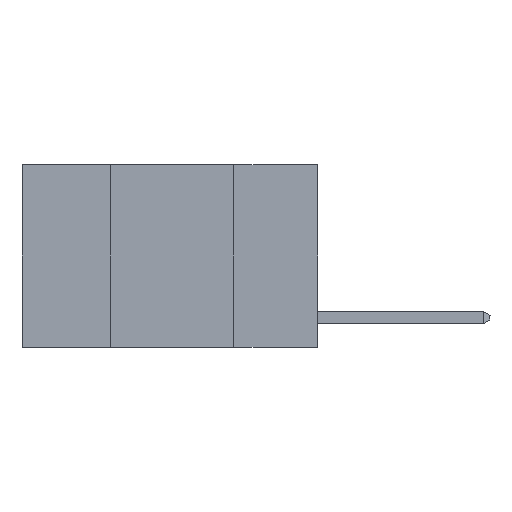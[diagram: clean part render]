
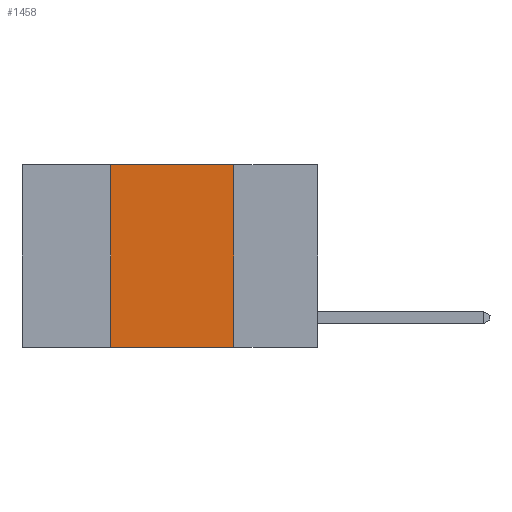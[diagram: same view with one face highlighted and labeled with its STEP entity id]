
A CAD part, left-side view. The second image highlights one B-rep face of the part: STEP entity #1458.
In plain terms, the highlighted planar face has unit normal (-1, 0, 0).
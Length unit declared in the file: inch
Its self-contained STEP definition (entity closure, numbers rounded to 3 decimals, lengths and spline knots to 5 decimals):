
#88 = LINE ( 'NONE', #13761, #22506 ) ;
#512 = VERTEX_POINT ( 'NONE', #4014 ) ;
#1458 = ADVANCED_FACE ( 'NONE', ( #5654 ), #13748, .F. ) ;
#1554 = DIRECTION ( 'NONE',  ( 0., 0., 1. ) ) ;
#3125 = EDGE_CURVE ( 'NONE', #16764, #26114, #20936, .T. ) ;
#3681 = DIRECTION ( 'NONE',  ( 0., -1., 0. ) ) ;
#4014 = CARTESIAN_POINT ( 'NONE',  ( 0., 0.42, -0.37 ) ) ;
#5654 = FACE_OUTER_BOUND ( 'NONE', #11573, .T. ) ;
#6169 = CARTESIAN_POINT ( 'NONE',  ( 0., 0.6, 0. ) ) ;
#6797 = EDGE_CURVE ( 'NONE', #25170, #16764, #20946, .T. ) ;
#6810 = DIRECTION ( 'NONE',  ( 1., 0., 0. ) ) ;
#7397 = CARTESIAN_POINT ( 'NONE',  ( 0., 0.17, -0.37 ) ) ;
#7670 = ORIENTED_EDGE ( 'NONE', *, *, #6797, .F. ) ;
#7905 = LINE ( 'NONE', #8155, #15253 ) ;
#8155 = CARTESIAN_POINT ( 'NONE',  ( 0., 0.42, 0. ) ) ;
#11036 = CARTESIAN_POINT ( 'NONE',  ( 0., 0.6, 0. ) ) ;
#11573 = EDGE_LOOP ( 'NONE', ( #22720, #7670, #16986, #24437 ) ) ;
#12397 = DIRECTION ( 'NONE',  ( 0., 0., -1. ) ) ;
#13748 = PLANE ( 'NONE',  #19317 ) ;
#13761 = CARTESIAN_POINT ( 'NONE',  ( 0., 0.6, -0.37 ) ) ;
#13836 = CARTESIAN_POINT ( 'NONE',  ( 0., 0.42, 0. ) ) ;
#14168 = EDGE_CURVE ( 'NONE', #512, #25170, #7905, .T. ) ;
#15253 = VECTOR ( 'NONE', #1554, 39.37008 ) ;
#16237 = VECTOR ( 'NONE', #25450, 39.37008 ) ;
#16619 = VECTOR ( 'NONE', #22917, 39.37008 ) ;
#16764 = VERTEX_POINT ( 'NONE', #24000 ) ;
#16981 = CARTESIAN_POINT ( 'NONE',  ( 0., 0.17, 0. ) ) ;
#16986 = ORIENTED_EDGE ( 'NONE', *, *, #14168, .F. ) ;
#19056 = EDGE_CURVE ( 'NONE', #512, #26114, #88, .T. ) ;
#19317 = AXIS2_PLACEMENT_3D ( 'NONE', #6169, #6810, #12397 ) ;
#20936 = LINE ( 'NONE', #16981, #16619 ) ;
#20946 = LINE ( 'NONE', #11036, #16237 ) ;
#22506 = VECTOR ( 'NONE', #3681, 39.37008 ) ;
#22720 = ORIENTED_EDGE ( 'NONE', *, *, #3125, .F. ) ;
#22917 = DIRECTION ( 'NONE',  ( 0., 0., -1. ) ) ;
#24000 = CARTESIAN_POINT ( 'NONE',  ( 0., 0.17, 0. ) ) ;
#24437 = ORIENTED_EDGE ( 'NONE', *, *, #19056, .T. ) ;
#25170 = VERTEX_POINT ( 'NONE', #13836 ) ;
#25450 = DIRECTION ( 'NONE',  ( 0., -1., 0. ) ) ;
#26114 = VERTEX_POINT ( 'NONE', #7397 ) ;
